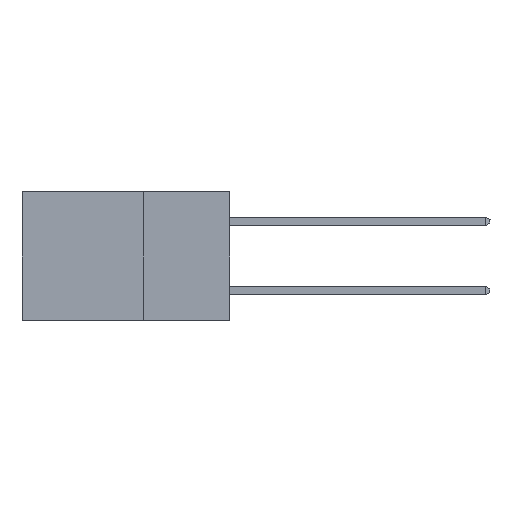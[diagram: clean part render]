
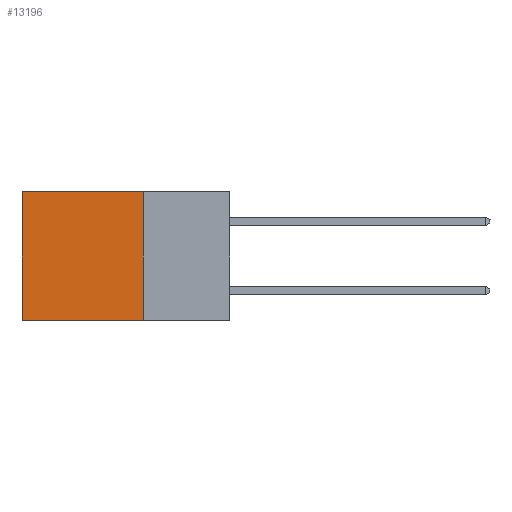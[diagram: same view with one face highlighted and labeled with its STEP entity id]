
A CAD part, left-side view. The second image highlights one B-rep face of the part: STEP entity #13196.
In plain terms, the highlighted planar face has unit normal (-1, 0, 0).
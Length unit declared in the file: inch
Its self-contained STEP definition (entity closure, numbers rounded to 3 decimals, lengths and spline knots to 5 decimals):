
#522 = EDGE_CURVE ( 'NONE', #15191, #12889, #2173, .T. ) ;
#1155 = ORIENTED_EDGE ( 'NONE', *, *, #15459, .T. ) ;
#1518 = CARTESIAN_POINT ( 'NONE',  ( 0.2615, 0.25, 0. ) ) ;
#2173 = LINE ( 'NONE', #17217, #16529 ) ;
#3983 = EDGE_CURVE ( 'NONE', #7481, #17428, #9824, .T. ) ;
#4599 = CARTESIAN_POINT ( 'NONE',  ( 0.2615, 0.25, -0.37 ) ) ;
#5125 = CARTESIAN_POINT ( 'NONE',  ( 0.2615, 0.25, -0.37 ) ) ;
#5622 = VECTOR ( 'NONE', #17484, 39.37008 ) ;
#5855 = DIRECTION ( 'NONE',  ( 0., 0., -1. ) ) ;
#6481 = DIRECTION ( 'NONE',  ( 0., 0., -1. ) ) ;
#6958 = DIRECTION ( 'NONE',  ( 0., 1., 0. ) ) ;
#7197 = CARTESIAN_POINT ( 'NONE',  ( 0.2615, 0.6, 0. ) ) ;
#7223 = EDGE_LOOP ( 'NONE', ( #10642, #8551, #10916, #1155 ) ) ;
#7481 = VERTEX_POINT ( 'NONE', #1518 ) ;
#8551 = ORIENTED_EDGE ( 'NONE', *, *, #15651, .F. ) ;
#9233 = VECTOR ( 'NONE', #6958, 39.37008 ) ;
#9824 = LINE ( 'NONE', #4599, #13972 ) ;
#10636 = DIRECTION ( 'NONE',  ( 1., 0., 0. ) ) ;
#10642 = ORIENTED_EDGE ( 'NONE', *, *, #522, .T. ) ;
#10916 = ORIENTED_EDGE ( 'NONE', *, *, #3983, .F. ) ;
#11981 = PLANE ( 'NONE',  #12093 ) ;
#11991 = LINE ( 'NONE', #17738, #5622 ) ;
#12084 = CARTESIAN_POINT ( 'NONE',  ( 0.2615, 0.25, -0.37 ) ) ;
#12093 = AXIS2_PLACEMENT_3D ( 'NONE', #5125, #10636, #6481 ) ;
#12200 = LINE ( 'NONE', #16426, #9233 ) ;
#12889 = VERTEX_POINT ( 'NONE', #16343 ) ;
#13196 = ADVANCED_FACE ( 'NONE', ( #17474 ), #11981, .F. ) ;
#13972 = VECTOR ( 'NONE', #5855, 39.37008 ) ;
#15191 = VERTEX_POINT ( 'NONE', #7197 ) ;
#15459 = EDGE_CURVE ( 'NONE', #7481, #15191, #12200, .T. ) ;
#15651 = EDGE_CURVE ( 'NONE', #17428, #12889, #11991, .T. ) ;
#15779 = DIRECTION ( 'NONE',  ( 0., 0., -1. ) ) ;
#16343 = CARTESIAN_POINT ( 'NONE',  ( 0.2615, 0.6, -0.37 ) ) ;
#16426 = CARTESIAN_POINT ( 'NONE',  ( 0.2615, 0.25, 0. ) ) ;
#16529 = VECTOR ( 'NONE', #15779, 39.37008 ) ;
#17217 = CARTESIAN_POINT ( 'NONE',  ( 0.2615, 0.6, -0.37 ) ) ;
#17428 = VERTEX_POINT ( 'NONE', #12084 ) ;
#17474 = FACE_OUTER_BOUND ( 'NONE', #7223, .T. ) ;
#17484 = DIRECTION ( 'NONE',  ( 0., 1., 0. ) ) ;
#17738 = CARTESIAN_POINT ( 'NONE',  ( 0.2615, 0.25, -0.37 ) ) ;
